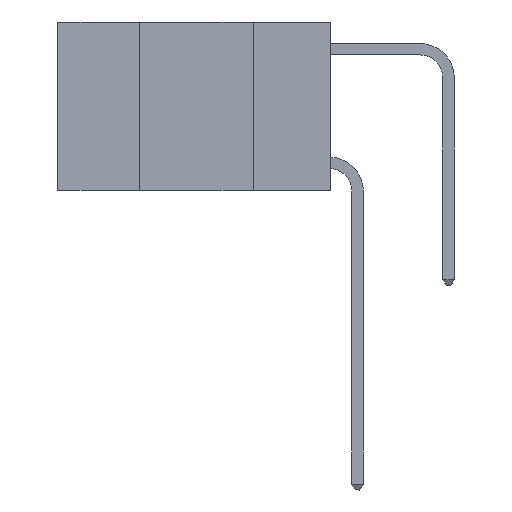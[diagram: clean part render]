
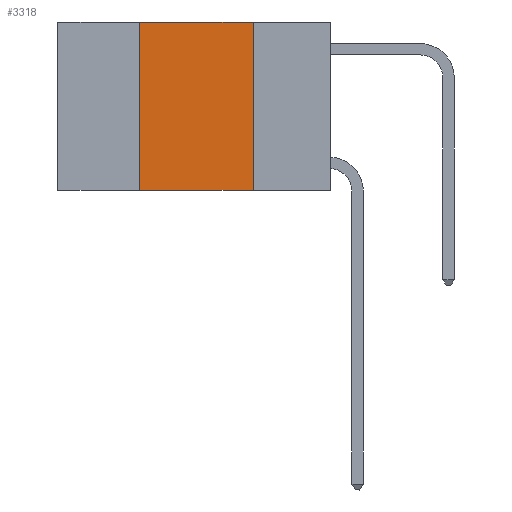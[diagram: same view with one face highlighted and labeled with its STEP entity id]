
A CAD part, left-side view. The second image highlights one B-rep face of the part: STEP entity #3318.
In plain terms, the highlighted planar face has unit normal (-1, 0, 0).
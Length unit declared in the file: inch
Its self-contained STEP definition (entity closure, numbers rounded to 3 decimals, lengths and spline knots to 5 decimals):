
#1276 = VERTEX_POINT ( 'NONE', #9076 ) ;
#1596 = CARTESIAN_POINT ( 'NONE',  ( 0., 0.6, 0. ) ) ;
#1685 = DIRECTION ( 'NONE',  ( 1., 0., 0. ) ) ;
#2007 = VECTOR ( 'NONE', #18287, 39.37008 ) ;
#3009 = PLANE ( 'NONE',  #7286 ) ;
#3259 = CARTESIAN_POINT ( 'NONE',  ( 0., 0.6, -0.37 ) ) ;
#3283 = VERTEX_POINT ( 'NONE', #15145 ) ;
#3318 = ADVANCED_FACE ( 'NONE', ( #12722 ), #3009, .F. ) ;
#3837 = CARTESIAN_POINT ( 'NONE',  ( 0., 0.6, 0. ) ) ;
#3903 = DIRECTION ( 'NONE',  ( 0., 0., 1. ) ) ;
#3984 = CARTESIAN_POINT ( 'NONE',  ( 0., 0.17, -0.37 ) ) ;
#4931 = VECTOR ( 'NONE', #15314, 39.37008 ) ;
#5835 = VECTOR ( 'NONE', #3903, 39.37008 ) ;
#6261 = ORIENTED_EDGE ( 'NONE', *, *, #10029, .F. ) ;
#6316 = EDGE_LOOP ( 'NONE', ( #8402, #6261, #20303, #23616 ) ) ;
#7286 = AXIS2_PLACEMENT_3D ( 'NONE', #1596, #1685, #13563 ) ;
#7957 = EDGE_CURVE ( 'NONE', #1276, #10395, #25216, .T. ) ;
#8402 = ORIENTED_EDGE ( 'NONE', *, *, #19306, .F. ) ;
#9076 = CARTESIAN_POINT ( 'NONE',  ( 0., 0.42, -0.37 ) ) ;
#10029 = EDGE_CURVE ( 'NONE', #3283, #12678, #22401, .T. ) ;
#10395 = VERTEX_POINT ( 'NONE', #3984 ) ;
#11985 = CARTESIAN_POINT ( 'NONE',  ( 0., 0.17, 0. ) ) ;
#12247 = CARTESIAN_POINT ( 'NONE',  ( 0., 0.42, 0. ) ) ;
#12678 = VERTEX_POINT ( 'NONE', #18371 ) ;
#12722 = FACE_OUTER_BOUND ( 'NONE', #6316, .T. ) ;
#13563 = DIRECTION ( 'NONE',  ( 0., 0., -1. ) ) ;
#15145 = CARTESIAN_POINT ( 'NONE',  ( 0., 0.42, 0. ) ) ;
#15314 = DIRECTION ( 'NONE',  ( 0., -1., 0. ) ) ;
#18287 = DIRECTION ( 'NONE',  ( 0., 0., -1. ) ) ;
#18371 = CARTESIAN_POINT ( 'NONE',  ( 0., 0.17, 0. ) ) ;
#19281 = EDGE_CURVE ( 'NONE', #1276, #3283, #24526, .T. ) ;
#19306 = EDGE_CURVE ( 'NONE', #12678, #10395, #20108, .T. ) ;
#20088 = DIRECTION ( 'NONE',  ( 0., -1., 0. ) ) ;
#20108 = LINE ( 'NONE', #11985, #2007 ) ;
#20303 = ORIENTED_EDGE ( 'NONE', *, *, #19281, .F. ) ;
#22401 = LINE ( 'NONE', #3837, #25515 ) ;
#23616 = ORIENTED_EDGE ( 'NONE', *, *, #7957, .T. ) ;
#24526 = LINE ( 'NONE', #12247, #5835 ) ;
#25216 = LINE ( 'NONE', #3259, #4931 ) ;
#25515 = VECTOR ( 'NONE', #20088, 39.37008 ) ;
